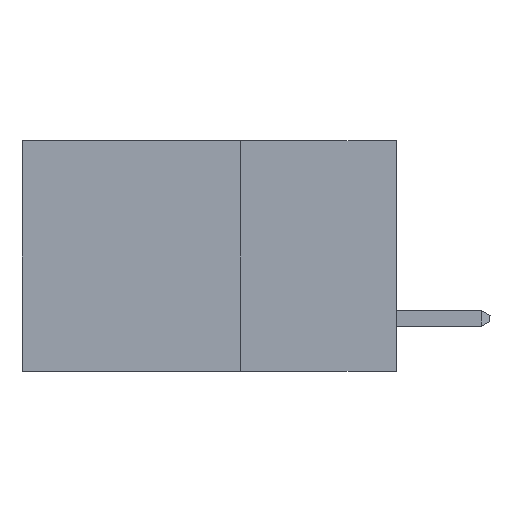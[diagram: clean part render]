
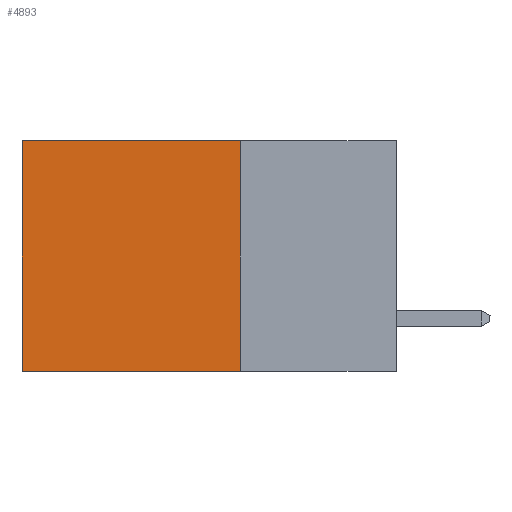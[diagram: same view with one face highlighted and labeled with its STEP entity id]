
A CAD part, left-side view. The second image highlights one B-rep face of the part: STEP entity #4893.
In plain terms, the highlighted planar face has unit normal (-1, 0, 0).
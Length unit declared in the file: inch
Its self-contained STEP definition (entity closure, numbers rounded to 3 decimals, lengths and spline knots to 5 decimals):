
#1690 = EDGE_CURVE ( 'NONE', #3972, #10544, #2630, .T. ) ;
#1803 = EDGE_CURVE ( 'NONE', #10544, #4902, #12498, .T. ) ;
#2042 = LINE ( 'NONE', #4429, #13235 ) ;
#2426 = EDGE_CURVE ( 'NONE', #2930, #4902, #13776, .T. ) ;
#2630 = LINE ( 'NONE', #12630, #10059 ) ;
#2930 = VERTEX_POINT ( 'NONE', #15168 ) ;
#3972 = VERTEX_POINT ( 'NONE', #5691 ) ;
#4036 = AXIS2_PLACEMENT_3D ( 'NONE', #16421, #14692, #14687 ) ;
#4429 = CARTESIAN_POINT ( 'NONE',  ( 0.2615, 0.25, -0.37 ) ) ;
#4893 = ADVANCED_FACE ( 'NONE', ( #9065 ), #15045, .F. ) ;
#4902 = VERTEX_POINT ( 'NONE', #14254 ) ;
#5382 = EDGE_LOOP ( 'NONE', ( #6620, #7804, #16243, #5399 ) ) ;
#5399 = ORIENTED_EDGE ( 'NONE', *, *, #1690, .T. ) ;
#5400 = DIRECTION ( 'NONE',  ( 0., 1., 0. ) ) ;
#5423 = CARTESIAN_POINT ( 'NONE',  ( 0.2615, 0.25, -0.37 ) ) ;
#5691 = CARTESIAN_POINT ( 'NONE',  ( 0.2615, 0.25, 0. ) ) ;
#5827 = DIRECTION ( 'NONE',  ( 0., 0., -1. ) ) ;
#6557 = VECTOR ( 'NONE', #5400, 39.37008 ) ;
#6620 = ORIENTED_EDGE ( 'NONE', *, *, #1803, .T. ) ;
#7130 = CARTESIAN_POINT ( 'NONE',  ( 0.2615, 0.6, 0. ) ) ;
#7804 = ORIENTED_EDGE ( 'NONE', *, *, #2426, .F. ) ;
#8161 = DIRECTION ( 'NONE',  ( 0., 1., 0. ) ) ;
#9065 = FACE_OUTER_BOUND ( 'NONE', #5382, .T. ) ;
#10059 = VECTOR ( 'NONE', #8161, 39.37008 ) ;
#10544 = VERTEX_POINT ( 'NONE', #7130 ) ;
#12053 = VECTOR ( 'NONE', #14359, 39.37008 ) ;
#12498 = LINE ( 'NONE', #17882, #12053 ) ;
#12630 = CARTESIAN_POINT ( 'NONE',  ( 0.2615, 0.25, 0. ) ) ;
#13235 = VECTOR ( 'NONE', #5827, 39.37008 ) ;
#13776 = LINE ( 'NONE', #5423, #6557 ) ;
#14254 = CARTESIAN_POINT ( 'NONE',  ( 0.2615, 0.6, -0.37 ) ) ;
#14359 = DIRECTION ( 'NONE',  ( 0., 0., -1. ) ) ;
#14610 = EDGE_CURVE ( 'NONE', #3972, #2930, #2042, .T. ) ;
#14687 = DIRECTION ( 'NONE',  ( 0., 0., -1. ) ) ;
#14692 = DIRECTION ( 'NONE',  ( 1., 0., 0. ) ) ;
#15045 = PLANE ( 'NONE',  #4036 ) ;
#15168 = CARTESIAN_POINT ( 'NONE',  ( 0.2615, 0.25, -0.37 ) ) ;
#16243 = ORIENTED_EDGE ( 'NONE', *, *, #14610, .F. ) ;
#16421 = CARTESIAN_POINT ( 'NONE',  ( 0.2615, 0.25, -0.37 ) ) ;
#17882 = CARTESIAN_POINT ( 'NONE',  ( 0.2615, 0.6, -0.37 ) ) ;
